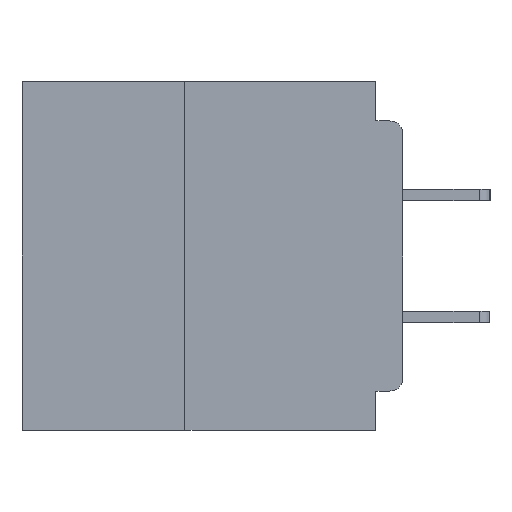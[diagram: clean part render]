
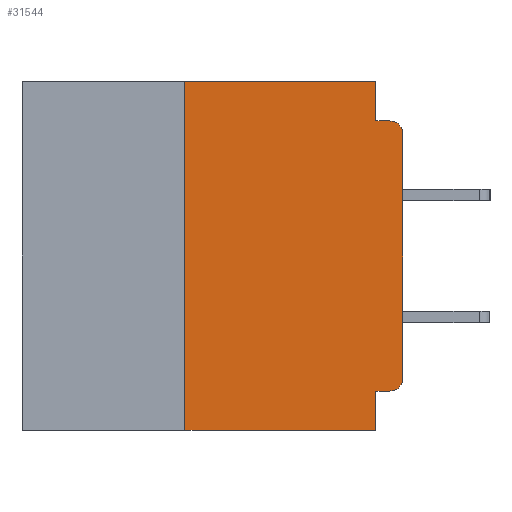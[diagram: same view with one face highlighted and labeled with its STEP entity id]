
A CAD part, left-side view. The second image highlights one B-rep face of the part: STEP entity #31544.
In plain terms, the highlighted planar face has unit normal (-1, 0, 0).
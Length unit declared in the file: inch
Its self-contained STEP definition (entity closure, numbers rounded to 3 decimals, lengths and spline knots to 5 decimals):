
#62 = ORIENTED_EDGE ( 'NONE', *, *, #23810, .T. ) ;
#224 = VERTEX_POINT ( 'NONE', #41415 ) ;
#406 = VERTEX_POINT ( 'NONE', #34581 ) ;
#483 = DIRECTION ( 'NONE',  ( 0., 0., -1. ) ) ;
#611 = LINE ( 'NONE', #21748, #40914 ) ;
#1642 = DIRECTION ( 'NONE',  ( 0., 0., -1. ) ) ;
#1821 = DIRECTION ( 'NONE',  ( 0., 0., -1. ) ) ;
#2533 = ORIENTED_EDGE ( 'NONE', *, *, #19590, .T. ) ;
#2722 = DIRECTION ( 'NONE',  ( 0., 0., -1. ) ) ;
#2911 = VECTOR ( 'NONE', #1821, 39.37008 ) ;
#5106 = EDGE_CURVE ( 'NONE', #406, #224, #18160, .T. ) ;
#5219 = CARTESIAN_POINT ( 'NONE',  ( 0., 0.031, -0.045 ) ) ;
#6606 = DIRECTION ( 'NONE',  ( 0., -1., 0. ) ) ;
#8007 = VECTOR ( 'NONE', #6606, 39.37008 ) ;
#8079 = LINE ( 'NONE', #28879, #48211 ) ;
#8448 = CARTESIAN_POINT ( 'NONE',  ( 0., 0.437, 0. ) ) ;
#8631 = DIRECTION ( 'NONE',  ( 0., -1., 0. ) ) ;
#9733 = EDGE_CURVE ( 'NONE', #224, #29002, #37569, .T. ) ;
#11431 = VERTEX_POINT ( 'NONE', #5219 ) ;
#11597 = ORIENTED_EDGE ( 'NONE', *, *, #28731, .F. ) ;
#11638 = AXIS2_PLACEMENT_3D ( 'NONE', #19820, #47771, #23845 ) ;
#11838 = EDGE_CURVE ( 'NONE', #47928, #49040, #31735, .T. ) ;
#12963 = CARTESIAN_POINT ( 'NONE',  ( 0., 0., -0.06 ) ) ;
#13396 = CARTESIAN_POINT ( 'NONE',  ( 0., 0.015, -0.355 ) ) ;
#13927 = CARTESIAN_POINT ( 'NONE',  ( 0., 0., -0.34 ) ) ;
#14250 = DIRECTION ( 'NONE',  ( 0., 0., 1. ) ) ;
#15185 = CIRCLE ( 'NONE', #47415, 0.015 ) ;
#16201 = VECTOR ( 'NONE', #20045, 39.37008 ) ;
#16222 = ORIENTED_EDGE ( 'NONE', *, *, #34538, .T. ) ;
#18160 = LINE ( 'NONE', #31504, #48807 ) ;
#18681 = CARTESIAN_POINT ( 'NONE',  ( 0., 0.031, 0. ) ) ;
#19590 = EDGE_CURVE ( 'NONE', #25970, #32794, #22386, .T. ) ;
#19820 = CARTESIAN_POINT ( 'NONE',  ( 0., 0.015, -0.06 ) ) ;
#20045 = DIRECTION ( 'NONE',  ( 0., -1., 0. ) ) ;
#21040 = VECTOR ( 'NONE', #27164, 39.37008 ) ;
#21648 = EDGE_CURVE ( 'NONE', #47928, #25970, #15185, .T. ) ;
#21748 = CARTESIAN_POINT ( 'NONE',  ( 0., 0.031, -0.4 ) ) ;
#21909 = CARTESIAN_POINT ( 'NONE',  ( 0., 0.031, 0. ) ) ;
#22386 = LINE ( 'NONE', #46150, #42428 ) ;
#23616 = EDGE_LOOP ( 'NONE', ( #2533, #62, #11597, #32897, #24032, #25634, #16222, #27163, #49746, #35008 ) ) ;
#23810 = EDGE_CURVE ( 'NONE', #32794, #41090, #28854, .T. ) ;
#23845 = DIRECTION ( 'NONE',  ( 0., 0., -1. ) ) ;
#24032 = ORIENTED_EDGE ( 'NONE', *, *, #9733, .F. ) ;
#24673 = DIRECTION ( 'NONE',  ( 1., 0., 0. ) ) ;
#25634 = ORIENTED_EDGE ( 'NONE', *, *, #5106, .F. ) ;
#25970 = VERTEX_POINT ( 'NONE', #13927 ) ;
#26823 = DIRECTION ( 'NONE',  ( -1., 0., 0. ) ) ;
#27163 = ORIENTED_EDGE ( 'NONE', *, *, #45695, .F. ) ;
#27164 = DIRECTION ( 'NONE',  ( 0., 1., 0. ) ) ;
#28731 = EDGE_CURVE ( 'NONE', #11431, #41090, #8079, .T. ) ;
#28854 = CIRCLE ( 'NONE', #11638, 0.015 ) ;
#28879 = CARTESIAN_POINT ( 'NONE',  ( 0., 0., -0.045 ) ) ;
#29002 = VERTEX_POINT ( 'NONE', #18681 ) ;
#29505 = CARTESIAN_POINT ( 'NONE',  ( 0., 0.031, -0.355 ) ) ;
#31110 = FACE_OUTER_BOUND ( 'NONE', #23616, .T. ) ;
#31504 = CARTESIAN_POINT ( 'NONE',  ( 0., 0.25, -0.4 ) ) ;
#31544 = ADVANCED_FACE ( 'NONE', ( #31110 ), #48590, .F. ) ;
#31735 = LINE ( 'NONE', #43096, #21040 ) ;
#32171 = CARTESIAN_POINT ( 'NONE',  ( 0., 0.437, -0.4 ) ) ;
#32418 = CARTESIAN_POINT ( 'NONE',  ( 0., 0.031, -0.4 ) ) ;
#32794 = VERTEX_POINT ( 'NONE', #12963 ) ;
#32897 = ORIENTED_EDGE ( 'NONE', *, *, #35025, .F. ) ;
#33201 = CARTESIAN_POINT ( 'NONE',  ( 0., 0.015, -0.045 ) ) ;
#34538 = EDGE_CURVE ( 'NONE', #406, #39975, #48132, .T. ) ;
#34581 = CARTESIAN_POINT ( 'NONE',  ( 0., 0.25, -0.4 ) ) ;
#34740 = CARTESIAN_POINT ( 'NONE',  ( 0., 0.437, 0. ) ) ;
#35008 = ORIENTED_EDGE ( 'NONE', *, *, #21648, .T. ) ;
#35025 = EDGE_CURVE ( 'NONE', #29002, #11431, #45592, .T. ) ;
#35097 = AXIS2_PLACEMENT_3D ( 'NONE', #8448, #24673, #483 ) ;
#37569 = LINE ( 'NONE', #34740, #8007 ) ;
#39537 = DIRECTION ( 'NONE',  ( 0., 0., 1. ) ) ;
#39975 = VERTEX_POINT ( 'NONE', #32418 ) ;
#40914 = VECTOR ( 'NONE', #1642, 39.37008 ) ;
#41090 = VERTEX_POINT ( 'NONE', #33201 ) ;
#41415 = CARTESIAN_POINT ( 'NONE',  ( 0., 0.25, 0. ) ) ;
#42428 = VECTOR ( 'NONE', #14250, 39.37008 ) ;
#43096 = CARTESIAN_POINT ( 'NONE',  ( 0., 0., -0.355 ) ) ;
#45592 = LINE ( 'NONE', #21909, #2911 ) ;
#45695 = EDGE_CURVE ( 'NONE', #49040, #39975, #611, .T. ) ;
#46150 = CARTESIAN_POINT ( 'NONE',  ( 0., 0., 0. ) ) ;
#47415 = AXIS2_PLACEMENT_3D ( 'NONE', #50728, #26823, #2722 ) ;
#47771 = DIRECTION ( 'NONE',  ( -1., 0., 0. ) ) ;
#47928 = VERTEX_POINT ( 'NONE', #13396 ) ;
#48132 = LINE ( 'NONE', #32171, #16201 ) ;
#48211 = VECTOR ( 'NONE', #8631, 39.37008 ) ;
#48590 = PLANE ( 'NONE',  #35097 ) ;
#48807 = VECTOR ( 'NONE', #39537, 39.37008 ) ;
#49040 = VERTEX_POINT ( 'NONE', #29505 ) ;
#49746 = ORIENTED_EDGE ( 'NONE', *, *, #11838, .F. ) ;
#50728 = CARTESIAN_POINT ( 'NONE',  ( 0., 0.015, -0.34 ) ) ;
